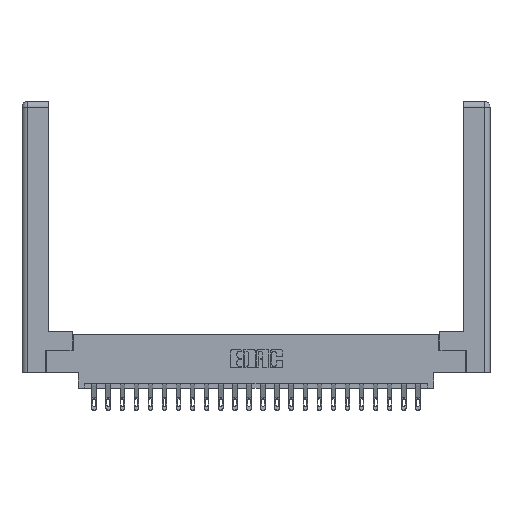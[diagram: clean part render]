
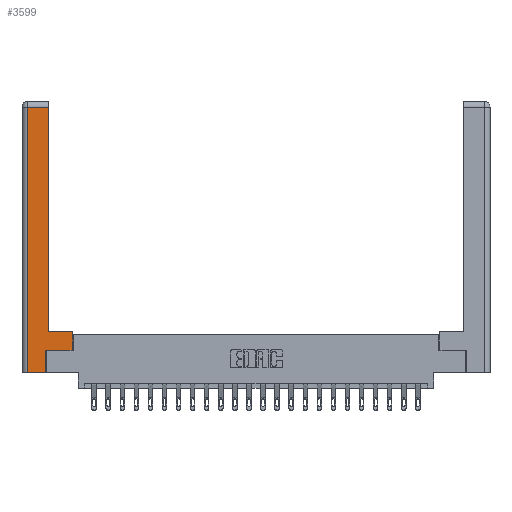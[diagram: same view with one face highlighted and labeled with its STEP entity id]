
A CAD part, top view. The second image highlights one B-rep face of the part: STEP entity #3599.
In plain terms, the highlighted planar face has unit normal (0, 0, 1).
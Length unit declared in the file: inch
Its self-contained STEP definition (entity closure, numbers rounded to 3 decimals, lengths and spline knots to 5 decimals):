
#404 = ORIENTED_EDGE ( 'NONE', *, *, #12142, .T. ) ;
#651 = VERTEX_POINT ( 'NONE', #8773 ) ;
#1364 = EDGE_CURVE ( 'NONE', #651, #2222, #15193, .T. ) ;
#1529 = EDGE_CURVE ( 'NONE', #6863, #12197, #20671, .T. ) ;
#1582 = VECTOR ( 'NONE', #19327, 39.37008 ) ;
#1626 = CARTESIAN_POINT ( 'NONE',  ( 0.295, 2.94, 0. ) ) ;
#2222 = VERTEX_POINT ( 'NONE', #5026 ) ;
#2289 = VERTEX_POINT ( 'NONE', #23703 ) ;
#2431 = LINE ( 'NONE', #4793, #14635 ) ;
#2582 = LINE ( 'NONE', #20856, #7499 ) ;
#3599 = ADVANCED_FACE ( 'NONE', ( #14838 ), #6488, .F. ) ;
#4193 = CARTESIAN_POINT ( 'NONE',  ( 0.565, 0.45, 0. ) ) ;
#4443 = VERTEX_POINT ( 'NONE', #21440 ) ;
#4520 = EDGE_CURVE ( 'NONE', #4443, #19573, #6073, .T. ) ;
#4595 = CARTESIAN_POINT ( 'NONE',  ( 0.0615, 0., 0. ) ) ;
#4793 = CARTESIAN_POINT ( 'NONE',  ( 0.565, 0.245, 0. ) ) ;
#5026 = CARTESIAN_POINT ( 'NONE',  ( 0.565, 0.45, 0. ) ) ;
#5367 = DIRECTION ( 'NONE',  ( 0., 1., 0. ) ) ;
#5496 = CARTESIAN_POINT ( 'NONE',  ( 0.0615, 2.94, 0. ) ) ;
#5585 = DIRECTION ( 'NONE',  ( 0., 1., 0. ) ) ;
#5732 = DIRECTION ( 'NONE',  ( -1., 0., 0. ) ) ;
#6073 = LINE ( 'NONE', #9145, #8375 ) ;
#6488 = PLANE ( 'NONE',  #15817 ) ;
#6643 = DIRECTION ( 'NONE',  ( 1., 0., 0. ) ) ;
#6863 = VERTEX_POINT ( 'NONE', #7050 ) ;
#7050 = CARTESIAN_POINT ( 'NONE',  ( 0.265, 0., 0. ) ) ;
#7499 = VECTOR ( 'NONE', #13313, 39.37008 ) ;
#8375 = VECTOR ( 'NONE', #5367, 39.37008 ) ;
#8499 = EDGE_LOOP ( 'NONE', ( #17685, #19567, #404, #11055, #13133, #22425, #21983, #13350 ) ) ;
#8773 = CARTESIAN_POINT ( 'NONE',  ( 0.565, 0.245, 0. ) ) ;
#9145 = CARTESIAN_POINT ( 'NONE',  ( 0.295, 3., 0. ) ) ;
#10193 = DIRECTION ( 'NONE',  ( -1., 0., 0. ) ) ;
#10209 = CARTESIAN_POINT ( 'NONE',  ( 0.0615, 0., 0. ) ) ;
#10389 = LINE ( 'NONE', #10209, #14196 ) ;
#11055 = ORIENTED_EDGE ( 'NONE', *, *, #18126, .T. ) ;
#12142 = EDGE_CURVE ( 'NONE', #2289, #12297, #10389, .T. ) ;
#12175 = DIRECTION ( 'NONE',  ( 0., 0., -1. ) ) ;
#12197 = VERTEX_POINT ( 'NONE', #15939 ) ;
#12274 = DIRECTION ( 'NONE',  ( 0., -1., 0. ) ) ;
#12297 = VERTEX_POINT ( 'NONE', #4595 ) ;
#12973 = EDGE_CURVE ( 'NONE', #2222, #4443, #2582, .T. ) ;
#13133 = ORIENTED_EDGE ( 'NONE', *, *, #1529, .T. ) ;
#13313 = DIRECTION ( 'NONE',  ( -1., 0., 0. ) ) ;
#13350 = ORIENTED_EDGE ( 'NONE', *, *, #12973, .T. ) ;
#13440 = VECTOR ( 'NONE', #5585, 39.37008 ) ;
#14196 = VECTOR ( 'NONE', #12274, 39.37008 ) ;
#14635 = VECTOR ( 'NONE', #6643, 39.37008 ) ;
#14838 = FACE_OUTER_BOUND ( 'NONE', #8499, .T. ) ;
#15193 = LINE ( 'NONE', #4193, #13440 ) ;
#15247 = EDGE_CURVE ( 'NONE', #19573, #2289, #18128, .T. ) ;
#15555 = CARTESIAN_POINT ( 'NONE',  ( 0.265, 0.245, 0. ) ) ;
#15817 = AXIS2_PLACEMENT_3D ( 'NONE', #19555, #12175, #10193 ) ;
#15819 = LINE ( 'NONE', #17451, #1582 ) ;
#15939 = CARTESIAN_POINT ( 'NONE',  ( 0.265, 0.245, 0. ) ) ;
#17219 = VECTOR ( 'NONE', #21305, 39.37008 ) ;
#17451 = CARTESIAN_POINT ( 'NONE',  ( 0.265, 0., 0. ) ) ;
#17546 = VECTOR ( 'NONE', #5732, 39.37008 ) ;
#17685 = ORIENTED_EDGE ( 'NONE', *, *, #4520, .T. ) ;
#18126 = EDGE_CURVE ( 'NONE', #12297, #6863, #15819, .T. ) ;
#18128 = LINE ( 'NONE', #5496, #17546 ) ;
#18373 = EDGE_CURVE ( 'NONE', #12197, #651, #2431, .T. ) ;
#19327 = DIRECTION ( 'NONE',  ( 1., 0., 0. ) ) ;
#19555 = CARTESIAN_POINT ( 'NONE',  ( 0., 0., 0. ) ) ;
#19567 = ORIENTED_EDGE ( 'NONE', *, *, #15247, .T. ) ;
#19573 = VERTEX_POINT ( 'NONE', #1626 ) ;
#20671 = LINE ( 'NONE', #15555, #17219 ) ;
#20856 = CARTESIAN_POINT ( 'NONE',  ( 0.295, 0.45, 0. ) ) ;
#21305 = DIRECTION ( 'NONE',  ( 0., 1., 0. ) ) ;
#21440 = CARTESIAN_POINT ( 'NONE',  ( 0.295, 0.45, 0. ) ) ;
#21983 = ORIENTED_EDGE ( 'NONE', *, *, #1364, .T. ) ;
#22425 = ORIENTED_EDGE ( 'NONE', *, *, #18373, .T. ) ;
#23703 = CARTESIAN_POINT ( 'NONE',  ( 0.0615, 2.94, 0. ) ) ;
